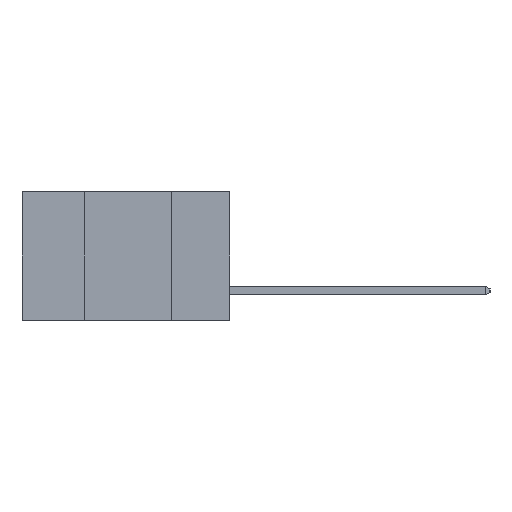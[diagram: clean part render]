
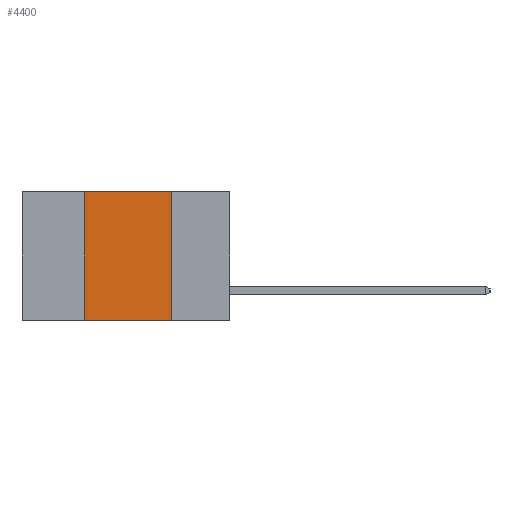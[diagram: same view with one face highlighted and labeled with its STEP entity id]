
A CAD part, left-side view. The second image highlights one B-rep face of the part: STEP entity #4400.
In plain terms, the highlighted planar face has unit normal (-1, 0, 0).
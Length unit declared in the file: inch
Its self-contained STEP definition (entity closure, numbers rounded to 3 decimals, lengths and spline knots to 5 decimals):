
#354 = EDGE_CURVE ( 'NONE', #8832, #19781, #18607, .T. ) ;
#2272 = DIRECTION ( 'NONE',  ( 1., 0., 0. ) ) ;
#2606 = EDGE_CURVE ( 'NONE', #10897, #8832, #7330, .T. ) ;
#2655 = VECTOR ( 'NONE', #16483, 39.37008 ) ;
#2845 = CARTESIAN_POINT ( 'NONE',  ( 0., 0.42, -0.37 ) ) ;
#3016 = DIRECTION ( 'NONE',  ( 0., 0., -1. ) ) ;
#3075 = VECTOR ( 'NONE', #19065, 39.37008 ) ;
#3668 = EDGE_CURVE ( 'NONE', #10897, #5942, #12572, .T. ) ;
#4400 = ADVANCED_FACE ( 'NONE', ( #7774 ), #11058, .F. ) ;
#4580 = ORIENTED_EDGE ( 'NONE', *, *, #17570, .F. ) ;
#5366 = EDGE_LOOP ( 'NONE', ( #4580, #20057, #20039, #17596 ) ) ;
#5781 = CARTESIAN_POINT ( 'NONE',  ( 0., 0.17, -0.37 ) ) ;
#5926 = AXIS2_PLACEMENT_3D ( 'NONE', #19095, #2272, #3016 ) ;
#5942 = VERTEX_POINT ( 'NONE', #5781 ) ;
#6050 = CARTESIAN_POINT ( 'NONE',  ( 0., 0.6, 0. ) ) ;
#7330 = LINE ( 'NONE', #2845, #3075 ) ;
#7774 = FACE_OUTER_BOUND ( 'NONE', #5366, .T. ) ;
#8832 = VERTEX_POINT ( 'NONE', #10043 ) ;
#9885 = CARTESIAN_POINT ( 'NONE',  ( 0., 0.42, -0.37 ) ) ;
#10041 = LINE ( 'NONE', #15452, #12172 ) ;
#10043 = CARTESIAN_POINT ( 'NONE',  ( 0., 0.42, 0. ) ) ;
#10897 = VERTEX_POINT ( 'NONE', #9885 ) ;
#11058 = PLANE ( 'NONE',  #5926 ) ;
#12172 = VECTOR ( 'NONE', #16959, 39.37008 ) ;
#12572 = LINE ( 'NONE', #14517, #19576 ) ;
#14318 = DIRECTION ( 'NONE',  ( 0., -1., 0. ) ) ;
#14517 = CARTESIAN_POINT ( 'NONE',  ( 0., 0.6, -0.37 ) ) ;
#15452 = CARTESIAN_POINT ( 'NONE',  ( 0., 0.17, -0.37 ) ) ;
#16483 = DIRECTION ( 'NONE',  ( 0., -1., 0. ) ) ;
#16959 = DIRECTION ( 'NONE',  ( 0., 0., -1. ) ) ;
#17570 = EDGE_CURVE ( 'NONE', #19781, #5942, #10041, .T. ) ;
#17596 = ORIENTED_EDGE ( 'NONE', *, *, #3668, .T. ) ;
#18607 = LINE ( 'NONE', #6050, #2655 ) ;
#19065 = DIRECTION ( 'NONE',  ( 0., 0., 1. ) ) ;
#19095 = CARTESIAN_POINT ( 'NONE',  ( 0., 0.6, 0. ) ) ;
#19576 = VECTOR ( 'NONE', #14318, 39.37008 ) ;
#19781 = VERTEX_POINT ( 'NONE', #19858 ) ;
#19858 = CARTESIAN_POINT ( 'NONE',  ( 0., 0.17, 0. ) ) ;
#20039 = ORIENTED_EDGE ( 'NONE', *, *, #2606, .F. ) ;
#20057 = ORIENTED_EDGE ( 'NONE', *, *, #354, .F. ) ;
